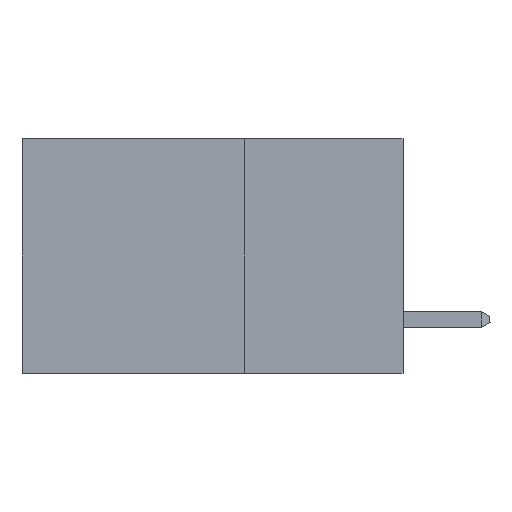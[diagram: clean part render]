
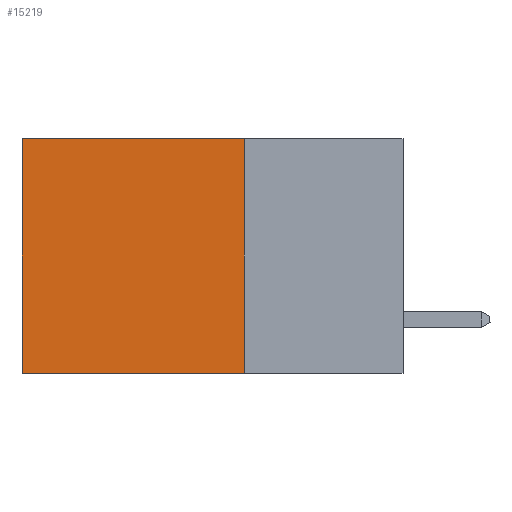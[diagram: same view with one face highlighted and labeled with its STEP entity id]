
A CAD part, left-side view. The second image highlights one B-rep face of the part: STEP entity #15219.
In plain terms, the highlighted planar face has unit normal (-1, 0, 0).
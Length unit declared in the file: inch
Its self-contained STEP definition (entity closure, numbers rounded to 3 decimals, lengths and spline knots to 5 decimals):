
#828 = CARTESIAN_POINT ( 'NONE',  ( 0.2875, 0.25, -0.37 ) ) ;
#1014 = LINE ( 'NONE', #11840, #12713 ) ;
#1330 = VECTOR ( 'NONE', #8452, 39.37008 ) ;
#2310 = CARTESIAN_POINT ( 'NONE',  ( 0.2875, 0.6, -0.37 ) ) ;
#2379 = DIRECTION ( 'NONE',  ( 0., 0., -1. ) ) ;
#2711 = VERTEX_POINT ( 'NONE', #16065 ) ;
#2740 = ORIENTED_EDGE ( 'NONE', *, *, #4628, .T. ) ;
#3088 = CARTESIAN_POINT ( 'NONE',  ( 0.2875, 0.25, 0. ) ) ;
#3334 = VERTEX_POINT ( 'NONE', #2310 ) ;
#3697 = EDGE_LOOP ( 'NONE', ( #15371, #17718, #15861, #2740 ) ) ;
#3771 = CARTESIAN_POINT ( 'NONE',  ( 0.2875, 0.25, 0. ) ) ;
#4628 = EDGE_CURVE ( 'NONE', #10651, #2711, #7629, .T. ) ;
#5284 = VECTOR ( 'NONE', #2379, 39.37008 ) ;
#5986 = CARTESIAN_POINT ( 'NONE',  ( 0.2875, 0.6, 0. ) ) ;
#6969 = PLANE ( 'NONE',  #18353 ) ;
#7629 = LINE ( 'NONE', #3771, #1330 ) ;
#8259 = CARTESIAN_POINT ( 'NONE',  ( 0.2875, 0.25, 0. ) ) ;
#8389 = DIRECTION ( 'NONE',  ( 0., 0., -1. ) ) ;
#8452 = DIRECTION ( 'NONE',  ( 0., 1., 0. ) ) ;
#9388 = CARTESIAN_POINT ( 'NONE',  ( 0.2875, 0.25, 0. ) ) ;
#9545 = VERTEX_POINT ( 'NONE', #828 ) ;
#9722 = DIRECTION ( 'NONE',  ( 1., 0., 0. ) ) ;
#10046 = DIRECTION ( 'NONE',  ( 0., 0., -1. ) ) ;
#10651 = VERTEX_POINT ( 'NONE', #3088 ) ;
#11840 = CARTESIAN_POINT ( 'NONE',  ( 0.2875, 0.25, -0.37 ) ) ;
#12713 = VECTOR ( 'NONE', #15868, 39.37008 ) ;
#12900 = LINE ( 'NONE', #5986, #18109 ) ;
#13175 = EDGE_CURVE ( 'NONE', #10651, #9545, #13412, .T. ) ;
#13412 = LINE ( 'NONE', #9388, #5284 ) ;
#15219 = ADVANCED_FACE ( 'NONE', ( #15480 ), #6969, .F. ) ;
#15371 = ORIENTED_EDGE ( 'NONE', *, *, #17236, .T. ) ;
#15480 = FACE_OUTER_BOUND ( 'NONE', #3697, .T. ) ;
#15861 = ORIENTED_EDGE ( 'NONE', *, *, #13175, .F. ) ;
#15868 = DIRECTION ( 'NONE',  ( 0., 1., 0. ) ) ;
#16027 = EDGE_CURVE ( 'NONE', #9545, #3334, #1014, .T. ) ;
#16065 = CARTESIAN_POINT ( 'NONE',  ( 0.2875, 0.6, 0. ) ) ;
#17236 = EDGE_CURVE ( 'NONE', #2711, #3334, #12900, .T. ) ;
#17718 = ORIENTED_EDGE ( 'NONE', *, *, #16027, .F. ) ;
#18109 = VECTOR ( 'NONE', #10046, 39.37008 ) ;
#18353 = AXIS2_PLACEMENT_3D ( 'NONE', #8259, #9722, #8389 ) ;
